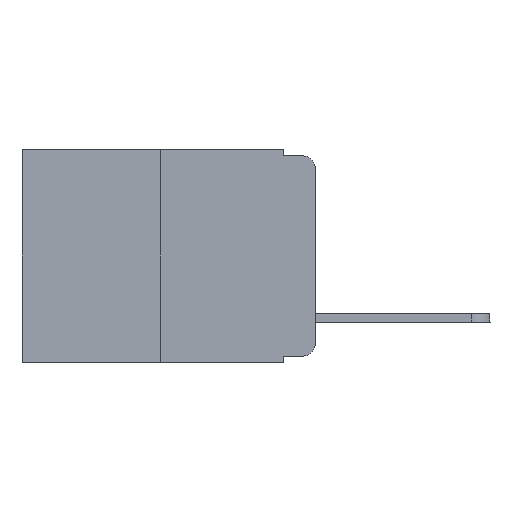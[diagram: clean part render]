
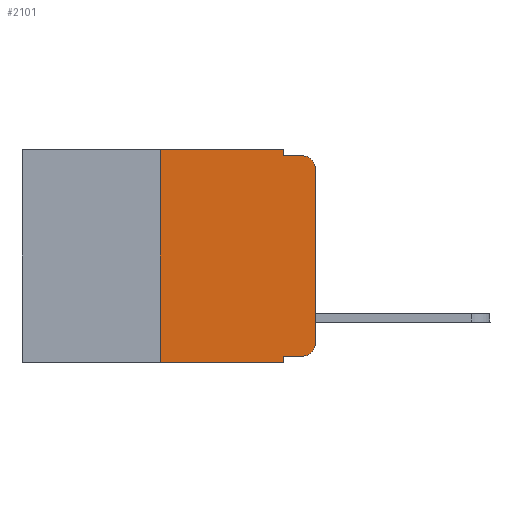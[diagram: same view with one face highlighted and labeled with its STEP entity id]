
A CAD part, left-side view. The second image highlights one B-rep face of the part: STEP entity #2101.
In plain terms, the highlighted planar face has unit normal (-1, 0, 0).
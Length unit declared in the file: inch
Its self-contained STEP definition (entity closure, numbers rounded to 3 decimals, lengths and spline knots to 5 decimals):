
#64 = EDGE_CURVE ( 'NONE', #6316, #2071, #8879, .T. ) ;
#133 = VECTOR ( 'NONE', #1272, 39.37008 ) ;
#157 = EDGE_CURVE ( 'NONE', #5296, #10501, #3859, .T. ) ;
#449 = LINE ( 'NONE', #11913, #4340 ) ;
#535 = CARTESIAN_POINT ( 'NONE',  ( 0., 0.051, -0.333 ) ) ;
#566 = CARTESIAN_POINT ( 'NONE',  ( 0., 0.25, -0.343 ) ) ;
#593 = CARTESIAN_POINT ( 'NONE',  ( 0., 0., -0.03 ) ) ;
#756 = ORIENTED_EDGE ( 'NONE', *, *, #6233, .F. ) ;
#1139 = DIRECTION ( 'NONE',  ( -1., 0., 0. ) ) ;
#1167 = VERTEX_POINT ( 'NONE', #7709 ) ;
#1192 = CARTESIAN_POINT ( 'NONE',  ( 0., 0.051, 0. ) ) ;
#1272 = DIRECTION ( 'NONE',  ( 0., 0., -1. ) ) ;
#1705 = ORIENTED_EDGE ( 'NONE', *, *, #11932, .F. ) ;
#1756 = CARTESIAN_POINT ( 'NONE',  ( 0., 0.473, 0. ) ) ;
#1973 = LINE ( 'NONE', #1192, #133 ) ;
#2011 = VECTOR ( 'NONE', #12448, 39.37008 ) ;
#2071 = VERTEX_POINT ( 'NONE', #6868 ) ;
#2101 = ADVANCED_FACE ( 'NONE', ( #7890 ), #10934, .F. ) ;
#2147 = CARTESIAN_POINT ( 'NONE',  ( 0., 0.25, 0. ) ) ;
#2367 = LINE ( 'NONE', #6211, #11755 ) ;
#2421 = ORIENTED_EDGE ( 'NONE', *, *, #6530, .F. ) ;
#2667 = LINE ( 'NONE', #10581, #6612 ) ;
#2956 = AXIS2_PLACEMENT_3D ( 'NONE', #8920, #8960, #6084 ) ;
#3064 = DIRECTION ( 'NONE',  ( 0., 0., -1. ) ) ;
#3859 = LINE ( 'NONE', #7356, #2011 ) ;
#3971 = CARTESIAN_POINT ( 'NONE',  ( 0., 0.473, 0. ) ) ;
#4197 = EDGE_CURVE ( 'NONE', #4804, #9349, #12414, .T. ) ;
#4242 = EDGE_CURVE ( 'NONE', #5296, #6316, #8368, .T. ) ;
#4340 = VECTOR ( 'NONE', #11875, 39.37008 ) ;
#4804 = VERTEX_POINT ( 'NONE', #11762 ) ;
#4840 = VERTEX_POINT ( 'NONE', #8787 ) ;
#5296 = VERTEX_POINT ( 'NONE', #566 ) ;
#5514 = DIRECTION ( 'NONE',  ( 0., 0., 1. ) ) ;
#5944 = DIRECTION ( 'NONE',  ( 0., 0., -1. ) ) ;
#6084 = DIRECTION ( 'NONE',  ( 0., 0., -1. ) ) ;
#6101 = EDGE_CURVE ( 'NONE', #9349, #6893, #8170, .T. ) ;
#6139 = ORIENTED_EDGE ( 'NONE', *, *, #64, .F. ) ;
#6211 = CARTESIAN_POINT ( 'NONE',  ( 0., 0.051, 0. ) ) ;
#6233 = EDGE_CURVE ( 'NONE', #2071, #1167, #2367, .T. ) ;
#6316 = VERTEX_POINT ( 'NONE', #2147 ) ;
#6530 = EDGE_CURVE ( 'NONE', #1167, #4840, #2667, .T. ) ;
#6567 = EDGE_LOOP ( 'NONE', ( #11744, #7866, #2421, #756, #6139, #10070, #6905, #1705, #8401, #8820 ) ) ;
#6612 = VECTOR ( 'NONE', #6703, 39.37008 ) ;
#6703 = DIRECTION ( 'NONE',  ( 0., -1., 0. ) ) ;
#6807 = VECTOR ( 'NONE', #5514, 39.37008 ) ;
#6868 = CARTESIAN_POINT ( 'NONE',  ( 0., 0.051, 0. ) ) ;
#6893 = VERTEX_POINT ( 'NONE', #12122 ) ;
#6905 = ORIENTED_EDGE ( 'NONE', *, *, #157, .T. ) ;
#7163 = VECTOR ( 'NONE', #8746, 39.37008 ) ;
#7356 = CARTESIAN_POINT ( 'NONE',  ( 0., 0.473, -0.343 ) ) ;
#7707 = VERTEX_POINT ( 'NONE', #593 ) ;
#7709 = CARTESIAN_POINT ( 'NONE',  ( 0., 0.051, -0.01 ) ) ;
#7866 = ORIENTED_EDGE ( 'NONE', *, *, #8740, .T. ) ;
#7890 = FACE_OUTER_BOUND ( 'NONE', #6567, .T. ) ;
#7990 = CARTESIAN_POINT ( 'NONE',  ( 0., 0.051, -0.343 ) ) ;
#8170 = CIRCLE ( 'NONE', #2956, 0.02 ) ;
#8368 = LINE ( 'NONE', #11493, #6807 ) ;
#8401 = ORIENTED_EDGE ( 'NONE', *, *, #4197, .T. ) ;
#8570 = EDGE_CURVE ( 'NONE', #6893, #7707, #449, .T. ) ;
#8740 = EDGE_CURVE ( 'NONE', #7707, #4840, #9305, .T. ) ;
#8746 = DIRECTION ( 'NONE',  ( 0., -1., 0. ) ) ;
#8787 = CARTESIAN_POINT ( 'NONE',  ( 0., 0.02, -0.01 ) ) ;
#8820 = ORIENTED_EDGE ( 'NONE', *, *, #6101, .T. ) ;
#8879 = LINE ( 'NONE', #1756, #7163 ) ;
#8920 = CARTESIAN_POINT ( 'NONE',  ( 0., 0.02, -0.313 ) ) ;
#8960 = DIRECTION ( 'NONE',  ( -1., 0., 0. ) ) ;
#9305 = CIRCLE ( 'NONE', #11470, 0.02 ) ;
#9349 = VERTEX_POINT ( 'NONE', #12856 ) ;
#10070 = ORIENTED_EDGE ( 'NONE', *, *, #4242, .F. ) ;
#10121 = CARTESIAN_POINT ( 'NONE',  ( 0., 0.02, -0.03 ) ) ;
#10194 = DIRECTION ( 'NONE',  ( 0., 0., -1. ) ) ;
#10274 = AXIS2_PLACEMENT_3D ( 'NONE', #3971, #11962, #5944 ) ;
#10501 = VERTEX_POINT ( 'NONE', #7990 ) ;
#10534 = DIRECTION ( 'NONE',  ( 0., -1., 0. ) ) ;
#10581 = CARTESIAN_POINT ( 'NONE',  ( 0., 0.051, -0.01 ) ) ;
#10862 = VECTOR ( 'NONE', #10534, 39.37008 ) ;
#10934 = PLANE ( 'NONE',  #10274 ) ;
#11470 = AXIS2_PLACEMENT_3D ( 'NONE', #10121, #1139, #3064 ) ;
#11493 = CARTESIAN_POINT ( 'NONE',  ( 0., 0.25, 0. ) ) ;
#11744 = ORIENTED_EDGE ( 'NONE', *, *, #8570, .T. ) ;
#11755 = VECTOR ( 'NONE', #10194, 39.37008 ) ;
#11762 = CARTESIAN_POINT ( 'NONE',  ( 0., 0.051, -0.333 ) ) ;
#11875 = DIRECTION ( 'NONE',  ( 0., 0., 1. ) ) ;
#11913 = CARTESIAN_POINT ( 'NONE',  ( 0., 0., 0. ) ) ;
#11932 = EDGE_CURVE ( 'NONE', #4804, #10501, #1973, .T. ) ;
#11962 = DIRECTION ( 'NONE',  ( 1., 0., 0. ) ) ;
#12122 = CARTESIAN_POINT ( 'NONE',  ( 0., 0., -0.313 ) ) ;
#12414 = LINE ( 'NONE', #535, #10862 ) ;
#12448 = DIRECTION ( 'NONE',  ( 0., -1., 0. ) ) ;
#12856 = CARTESIAN_POINT ( 'NONE',  ( 0., 0.02, -0.333 ) ) ;
